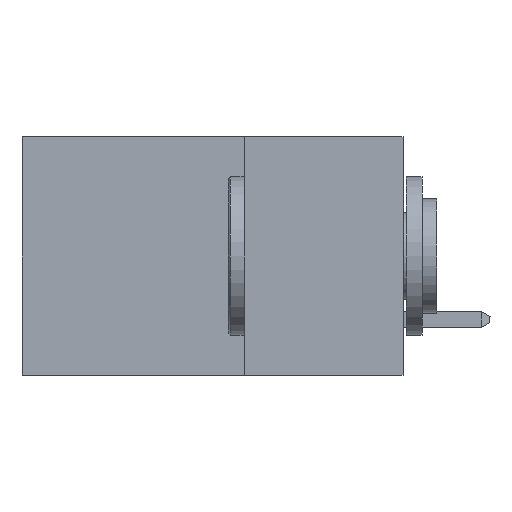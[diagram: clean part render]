
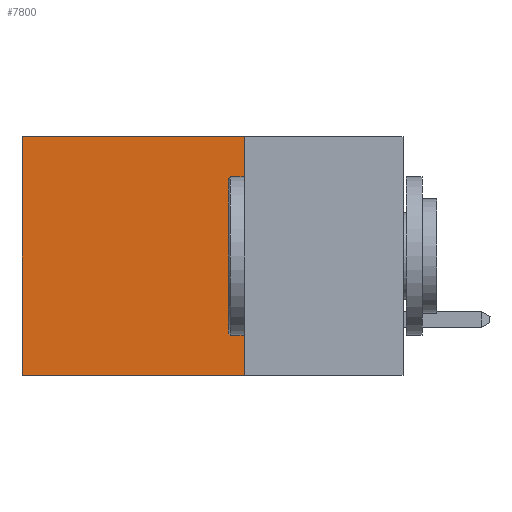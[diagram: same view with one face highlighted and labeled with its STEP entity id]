
A CAD part, left-side view. The second image highlights one B-rep face of the part: STEP entity #7800.
In plain terms, the highlighted planar face has unit normal (-1, 0, 0).
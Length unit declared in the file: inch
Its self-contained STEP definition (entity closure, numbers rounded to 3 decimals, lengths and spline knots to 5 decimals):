
#39 = ORIENTED_EDGE ( 'NONE', *, *, #6716, .T. ) ;
#183 = CARTESIAN_POINT ( 'NONE',  ( 0.2875, 0.25, -0.375 ) ) ;
#1144 = DIRECTION ( 'NONE',  ( 0., 0., -1. ) ) ;
#1225 = CARTESIAN_POINT ( 'NONE',  ( 0.2875, 0.25, 0. ) ) ;
#1344 = ORIENTED_EDGE ( 'NONE', *, *, #3249, .F. ) ;
#1401 = VERTEX_POINT ( 'NONE', #8092 ) ;
#1417 = VERTEX_POINT ( 'NONE', #3325 ) ;
#1621 = EDGE_CURVE ( 'NONE', #1401, #1417, #8652, .T. ) ;
#1765 = DIRECTION ( 'NONE',  ( 0., 0., -1. ) ) ;
#1918 = CARTESIAN_POINT ( 'NONE',  ( 0.2875, 0.25, -0.375 ) ) ;
#2083 = VECTOR ( 'NONE', #2930, 39.37008 ) ;
#2087 = EDGE_CURVE ( 'NONE', #3628, #4875, #4850, .T. ) ;
#2698 = CARTESIAN_POINT ( 'NONE',  ( 0.2875, 0.25, -0.375 ) ) ;
#2930 = DIRECTION ( 'NONE',  ( 0., 1., 0. ) ) ;
#3249 = EDGE_CURVE ( 'NONE', #4875, #1417, #5432, .T. ) ;
#3297 = DIRECTION ( 'NONE',  ( 0., 0., -1. ) ) ;
#3325 = CARTESIAN_POINT ( 'NONE',  ( 0.2875, 0.6, -0.375 ) ) ;
#3398 = LINE ( 'NONE', #6780, #5567 ) ;
#3628 = VERTEX_POINT ( 'NONE', #1225 ) ;
#4211 = VECTOR ( 'NONE', #1765, 39.37008 ) ;
#4476 = FACE_OUTER_BOUND ( 'NONE', #4553, .T. ) ;
#4553 = EDGE_LOOP ( 'NONE', ( #5661, #1344, #8225, #39 ) ) ;
#4764 = DIRECTION ( 'NONE',  ( 1., 0., 0. ) ) ;
#4850 = LINE ( 'NONE', #5290, #7664 ) ;
#4875 = VERTEX_POINT ( 'NONE', #2698 ) ;
#5290 = CARTESIAN_POINT ( 'NONE',  ( 0.2875, 0.25, -0.375 ) ) ;
#5432 = LINE ( 'NONE', #183, #2083 ) ;
#5567 = VECTOR ( 'NONE', #6020, 39.37008 ) ;
#5661 = ORIENTED_EDGE ( 'NONE', *, *, #1621, .T. ) ;
#5917 = AXIS2_PLACEMENT_3D ( 'NONE', #1918, #4764, #3297 ) ;
#6020 = DIRECTION ( 'NONE',  ( 0., 1., 0. ) ) ;
#6055 = PLANE ( 'NONE',  #5917 ) ;
#6716 = EDGE_CURVE ( 'NONE', #3628, #1401, #3398, .T. ) ;
#6780 = CARTESIAN_POINT ( 'NONE',  ( 0.2875, 0.25, 0. ) ) ;
#7294 = CARTESIAN_POINT ( 'NONE',  ( 0.2875, 0.6, -0.375 ) ) ;
#7664 = VECTOR ( 'NONE', #1144, 39.37008 ) ;
#7800 = ADVANCED_FACE ( 'NONE', ( #4476 ), #6055, .F. ) ;
#8092 = CARTESIAN_POINT ( 'NONE',  ( 0.2875, 0.6, 0. ) ) ;
#8225 = ORIENTED_EDGE ( 'NONE', *, *, #2087, .F. ) ;
#8652 = LINE ( 'NONE', #7294, #4211 ) ;
